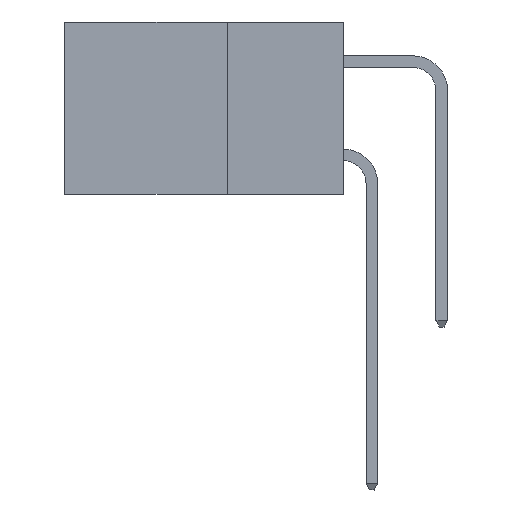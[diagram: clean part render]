
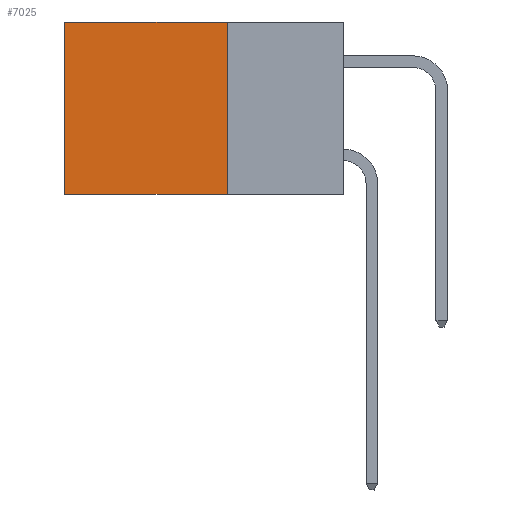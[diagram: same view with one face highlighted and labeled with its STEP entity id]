
A CAD part, left-side view. The second image highlights one B-rep face of the part: STEP entity #7025.
In plain terms, the highlighted planar face has unit normal (-1, 0, 0).
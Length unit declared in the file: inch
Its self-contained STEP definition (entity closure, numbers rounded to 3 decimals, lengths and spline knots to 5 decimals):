
#1361 = ORIENTED_EDGE ( 'NONE', *, *, #10227, .T. ) ;
#1968 = DIRECTION ( 'NONE',  ( 1., 0., 0. ) ) ;
#2179 = CARTESIAN_POINT ( 'NONE',  ( 0.2615, 0.25, -0.37 ) ) ;
#4168 = CARTESIAN_POINT ( 'NONE',  ( 0.2615, 0.25, -0.37 ) ) ;
#5607 = LINE ( 'NONE', #6055, #21783 ) ;
#6055 = CARTESIAN_POINT ( 'NONE',  ( 0.2615, 0.6, -0.37 ) ) ;
#6934 = CARTESIAN_POINT ( 'NONE',  ( 0.2615, 0.25, -0.37 ) ) ;
#7025 = ADVANCED_FACE ( 'NONE', ( #29188 ), #22332, .F. ) ;
#7112 = EDGE_LOOP ( 'NONE', ( #1361, #10740, #13719, #10347 ) ) ;
#9049 = CARTESIAN_POINT ( 'NONE',  ( 0.2615, 0.6, -0.37 ) ) ;
#9060 = VERTEX_POINT ( 'NONE', #9049 ) ;
#10227 = EDGE_CURVE ( 'NONE', #12353, #9060, #5607, .T. ) ;
#10347 = ORIENTED_EDGE ( 'NONE', *, *, #23986, .T. ) ;
#10495 = EDGE_CURVE ( 'NONE', #15339, #9060, #27322, .T. ) ;
#10740 = ORIENTED_EDGE ( 'NONE', *, *, #10495, .F. ) ;
#11363 = VECTOR ( 'NONE', #11847, 39.37008 ) ;
#11847 = DIRECTION ( 'NONE',  ( 0., 1., 0. ) ) ;
#12353 = VERTEX_POINT ( 'NONE', #19527 ) ;
#13719 = ORIENTED_EDGE ( 'NONE', *, *, #18698, .F. ) ;
#14509 = CARTESIAN_POINT ( 'NONE',  ( 0.2615, 0.25, 0. ) ) ;
#15115 = DIRECTION ( 'NONE',  ( 0., 0., -1. ) ) ;
#15160 = VERTEX_POINT ( 'NONE', #14509 ) ;
#15339 = VERTEX_POINT ( 'NONE', #2179 ) ;
#16471 = CARTESIAN_POINT ( 'NONE',  ( 0.2615, 0.25, 0. ) ) ;
#18698 = EDGE_CURVE ( 'NONE', #15160, #15339, #24255, .T. ) ;
#18731 = LINE ( 'NONE', #16471, #23285 ) ;
#19527 = CARTESIAN_POINT ( 'NONE',  ( 0.2615, 0.6, 0. ) ) ;
#19957 = CARTESIAN_POINT ( 'NONE',  ( 0.2615, 0.25, -0.37 ) ) ;
#20792 = DIRECTION ( 'NONE',  ( 0., 1., 0. ) ) ;
#21024 = VECTOR ( 'NONE', #22305, 39.37008 ) ;
#21783 = VECTOR ( 'NONE', #15115, 39.37008 ) ;
#22305 = DIRECTION ( 'NONE',  ( 0., 0., -1. ) ) ;
#22332 = PLANE ( 'NONE',  #29283 ) ;
#23285 = VECTOR ( 'NONE', #20792, 39.37008 ) ;
#23986 = EDGE_CURVE ( 'NONE', #15160, #12353, #18731, .T. ) ;
#24255 = LINE ( 'NONE', #4168, #21024 ) ;
#24861 = DIRECTION ( 'NONE',  ( 0., 0., -1. ) ) ;
#27322 = LINE ( 'NONE', #6934, #11363 ) ;
#29188 = FACE_OUTER_BOUND ( 'NONE', #7112, .T. ) ;
#29283 = AXIS2_PLACEMENT_3D ( 'NONE', #19957, #1968, #24861 ) ;
